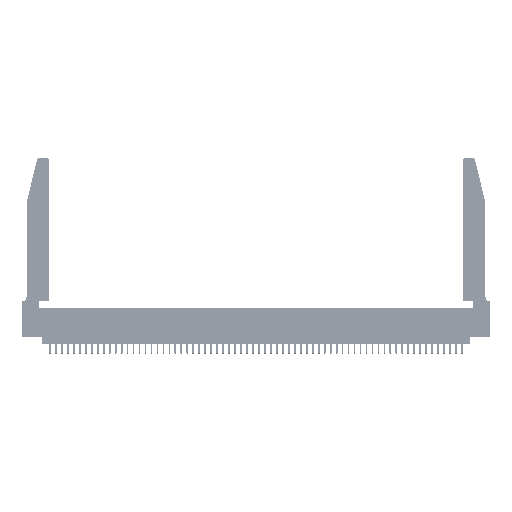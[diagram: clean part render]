
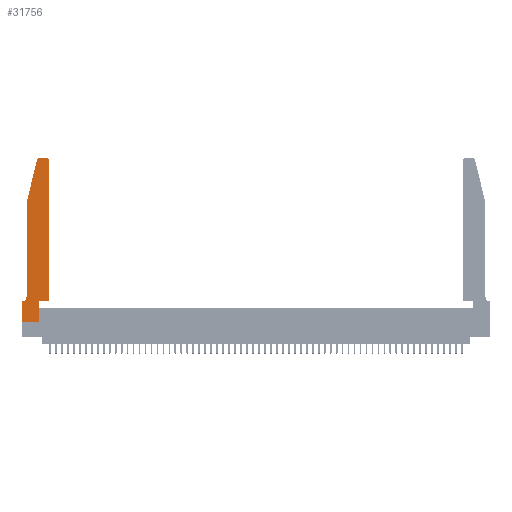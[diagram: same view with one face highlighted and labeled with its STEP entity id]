
A CAD part, top view. The second image highlights one B-rep face of the part: STEP entity #31756.
In plain terms, the highlighted planar face has unit normal (0, 0, 1).
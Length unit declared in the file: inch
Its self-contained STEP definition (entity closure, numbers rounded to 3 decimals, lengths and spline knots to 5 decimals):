
#1692 = AXIS2_PLACEMENT_3D ( 'NONE', #21656, #8760, #48019 ) ;
#1711 = VECTOR ( 'NONE', #22924, 39.37008 ) ;
#1972 = VERTEX_POINT ( 'NONE', #28880 ) ;
#2383 = CARTESIAN_POINT ( 'NONE',  ( 0., 0., 0.37 ) ) ;
#2435 = EDGE_CURVE ( 'NONE', #1972, #50223, #2860, .T. ) ;
#2860 = LINE ( 'NONE', #47074, #36742 ) ;
#3186 = DIRECTION ( 'NONE',  ( -1., 0., 0. ) ) ;
#3369 = CARTESIAN_POINT ( 'NONE',  ( 0.0055, 0.42, 0.37 ) ) ;
#4545 = DIRECTION ( 'NONE',  ( -1., 0., 0. ) ) ;
#5173 = LINE ( 'NONE', #23030, #11237 ) ;
#5466 = ORIENTED_EDGE ( 'NONE', *, *, #32638, .T. ) ;
#5831 = EDGE_CURVE ( 'NONE', #21304, #26186, #22012, .T. ) ;
#6552 = EDGE_CURVE ( 'NONE', #37347, #42776, #19202, .T. ) ;
#7027 = CARTESIAN_POINT ( 'NONE',  ( 0.4505, 0.35, 0.37 ) ) ;
#7184 = DIRECTION ( 'NONE',  ( 0., 1., 0. ) ) ;
#8057 = DIRECTION ( 'NONE',  ( 1., 0., 0. ) ) ;
#8760 = DIRECTION ( 'NONE',  ( 0., 0., 1. ) ) ;
#9457 = VERTEX_POINT ( 'NONE', #39178 ) ;
#11237 = VECTOR ( 'NONE', #13743, 39.37008 ) ;
#12635 = DIRECTION ( 'NONE',  ( 1., 0., 0. ) ) ;
#12733 = CIRCLE ( 'NONE', #1692, 0.03 ) ;
#13256 = ORIENTED_EDGE ( 'NONE', *, *, #16743, .T. ) ;
#13454 = ORIENTED_EDGE ( 'NONE', *, *, #31535, .T. ) ;
#13743 = DIRECTION ( 'NONE',  ( -0.239, -0.971, 0. ) ) ;
#14000 = ORIENTED_EDGE ( 'NONE', *, *, #6552, .T. ) ;
#14223 = CARTESIAN_POINT ( 'NONE',  ( 0.4205, 2.75, 0.37 ) ) ;
#16296 = DIRECTION ( 'NONE',  ( 1., 0., 0. ) ) ;
#16743 = EDGE_CURVE ( 'NONE', #45952, #26872, #46743, .T. ) ;
#16918 = EDGE_CURVE ( 'NONE', #42776, #46693, #48033, .T. ) ;
#17185 = CARTESIAN_POINT ( 'NONE',  ( 0.4505, 2.72, 0.37 ) ) ;
#17517 = DIRECTION ( 'NONE',  ( 0., 0., 1. ) ) ;
#17680 = FACE_OUTER_BOUND ( 'NONE', #50934, .T. ) ;
#19202 = CIRCLE ( 'NONE', #26384, 0.03 ) ;
#19446 = CARTESIAN_POINT ( 'NONE',  ( 0.0055, 0.35, 0.37 ) ) ;
#19769 = CIRCLE ( 'NONE', #49201, 0.07 ) ;
#20071 = CARTESIAN_POINT ( 'NONE',  ( 0.2865, 0., 0.37 ) ) ;
#21059 = DIRECTION ( 'NONE',  ( 0., -1., 0. ) ) ;
#21304 = VERTEX_POINT ( 'NONE', #19446 ) ;
#21309 = CARTESIAN_POINT ( 'NONE',  ( 0., 0., 0.37 ) ) ;
#21498 = EDGE_CURVE ( 'NONE', #28550, #45952, #46921, .T. ) ;
#21574 = CARTESIAN_POINT ( 'NONE',  ( 0.2605, 2.75, 0.37 ) ) ;
#21656 = CARTESIAN_POINT ( 'NONE',  ( 0.284, 2.72, 0.37 ) ) ;
#21979 = CARTESIAN_POINT ( 'NONE',  ( 0.0755, 0.35, 0.37 ) ) ;
#22012 = LINE ( 'NONE', #21979, #1711 ) ;
#22126 = ORIENTED_EDGE ( 'NONE', *, *, #27386, .T. ) ;
#22346 = VECTOR ( 'NONE', #7184, 39.37008 ) ;
#22512 = VECTOR ( 'NONE', #44361, 39.37008 ) ;
#22879 = DIRECTION ( 'NONE',  ( 0., 0., 1. ) ) ;
#22924 = DIRECTION ( 'NONE',  ( -1., 0., 0. ) ) ;
#23030 = CARTESIAN_POINT ( 'NONE',  ( 0.0755, 2., 0.37 ) ) ;
#23541 = ORIENTED_EDGE ( 'NONE', *, *, #16918, .T. ) ;
#23768 = VECTOR ( 'NONE', #16296, 39.37008 ) ;
#24759 = DIRECTION ( 'NONE',  ( 0., 0., -1. ) ) ;
#26186 = VERTEX_POINT ( 'NONE', #31175 ) ;
#26384 = AXIS2_PLACEMENT_3D ( 'NONE', #30778, #17517, #52482 ) ;
#26872 = VERTEX_POINT ( 'NONE', #40360 ) ;
#27137 = LINE ( 'NONE', #7027, #23768 ) ;
#27292 = LINE ( 'NONE', #36195, #22512 ) ;
#27386 = EDGE_CURVE ( 'NONE', #9457, #37347, #36593, .T. ) ;
#28550 = VERTEX_POINT ( 'NONE', #2383 ) ;
#28880 = CARTESIAN_POINT ( 'NONE',  ( 0.0755, 2., 0.37 ) ) ;
#29628 = VERTEX_POINT ( 'NONE', #36167 ) ;
#30778 = CARTESIAN_POINT ( 'NONE',  ( 0.4205, 2.72, 0.37 ) ) ;
#31175 = CARTESIAN_POINT ( 'NONE',  ( 0., 0.35, 0.37 ) ) ;
#31255 = ORIENTED_EDGE ( 'NONE', *, *, #2435, .T. ) ;
#31535 = EDGE_CURVE ( 'NONE', #50223, #21304, #19769, .T. ) ;
#31756 = ADVANCED_FACE ( 'NONE', ( #17680 ), #48885, .T. ) ;
#32094 = ORIENTED_EDGE ( 'NONE', *, *, #36295, .T. ) ;
#32250 = ORIENTED_EDGE ( 'NONE', *, *, #42851, .T. ) ;
#32638 = EDGE_CURVE ( 'NONE', #26872, #9457, #27137, .T. ) ;
#35180 = VECTOR ( 'NONE', #51029, 39.37008 ) ;
#36167 = CARTESIAN_POINT ( 'NONE',  ( 0.25487, 2.72718, 0.37 ) ) ;
#36195 = CARTESIAN_POINT ( 'NONE',  ( 0., 0., 0.37 ) ) ;
#36295 = EDGE_CURVE ( 'NONE', #29628, #1972, #5173, .T. ) ;
#36494 = VECTOR ( 'NONE', #4545, 39.37008 ) ;
#36593 = LINE ( 'NONE', #37715, #22346 ) ;
#36742 = VECTOR ( 'NONE', #21059, 39.37008 ) ;
#37347 = VERTEX_POINT ( 'NONE', #17185 ) ;
#37715 = CARTESIAN_POINT ( 'NONE',  ( 0.4505, 0.35, 0.37 ) ) ;
#39178 = CARTESIAN_POINT ( 'NONE',  ( 0.4505, 0.35, 0.37 ) ) ;
#40360 = CARTESIAN_POINT ( 'NONE',  ( 0.2865, 0.35, 0.37 ) ) ;
#42776 = VERTEX_POINT ( 'NONE', #14223 ) ;
#42851 = EDGE_CURVE ( 'NONE', #26186, #28550, #27292, .T. ) ;
#43320 = ORIENTED_EDGE ( 'NONE', *, *, #21498, .T. ) ;
#44118 = CARTESIAN_POINT ( 'NONE',  ( 0., 0.35, 0.37 ) ) ;
#44361 = DIRECTION ( 'NONE',  ( 0., -1., 0. ) ) ;
#45532 = EDGE_CURVE ( 'NONE', #46693, #29628, #12733, .T. ) ;
#45952 = VERTEX_POINT ( 'NONE', #20071 ) ;
#46693 = VERTEX_POINT ( 'NONE', #47355 ) ;
#46743 = LINE ( 'NONE', #55400, #35180 ) ;
#46921 = LINE ( 'NONE', #21309, #47565 ) ;
#47074 = CARTESIAN_POINT ( 'NONE',  ( 0.0755, 2., 0.37 ) ) ;
#47355 = CARTESIAN_POINT ( 'NONE',  ( 0.284, 2.75, 0.37 ) ) ;
#47356 = AXIS2_PLACEMENT_3D ( 'NONE', #44118, #22879, #12635 ) ;
#47565 = VECTOR ( 'NONE', #8057, 39.37008 ) ;
#48019 = DIRECTION ( 'NONE',  ( 1., 0., 0. ) ) ;
#48033 = LINE ( 'NONE', #21574, #36494 ) ;
#48885 = PLANE ( 'NONE',  #47356 ) ;
#49201 = AXIS2_PLACEMENT_3D ( 'NONE', #3369, #24759, #3186 ) ;
#50223 = VERTEX_POINT ( 'NONE', #52478 ) ;
#50934 = EDGE_LOOP ( 'NONE', ( #23541, #55509, #32094, #31255, #13454, #51697, #32250, #43320, #13256, #5466, #22126, #14000 ) ) ;
#51029 = DIRECTION ( 'NONE',  ( 0., 1., 0. ) ) ;
#51697 = ORIENTED_EDGE ( 'NONE', *, *, #5831, .T. ) ;
#52478 = CARTESIAN_POINT ( 'NONE',  ( 0.0755, 0.42, 0.37 ) ) ;
#52482 = DIRECTION ( 'NONE',  ( 1., 0., 0. ) ) ;
#55400 = CARTESIAN_POINT ( 'NONE',  ( 0.2865, 0.35, 0.37 ) ) ;
#55509 = ORIENTED_EDGE ( 'NONE', *, *, #45532, .T. ) ;
